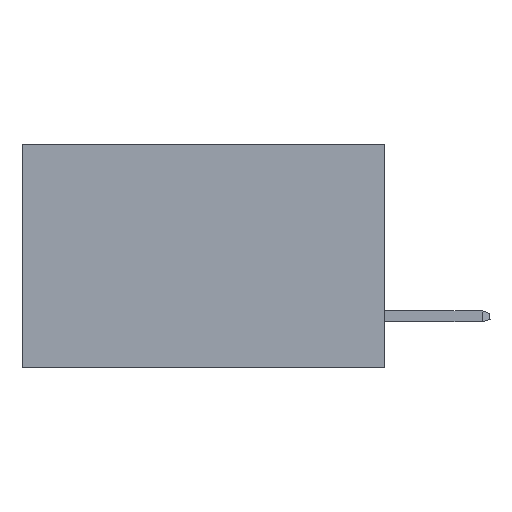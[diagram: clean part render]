
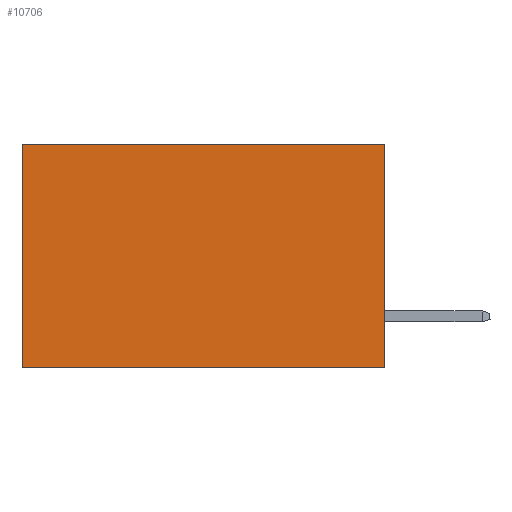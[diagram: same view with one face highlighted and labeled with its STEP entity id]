
A CAD part, left-side view. The second image highlights one B-rep face of the part: STEP entity #10706.
In plain terms, the highlighted planar face has unit normal (-1, 0, 0).
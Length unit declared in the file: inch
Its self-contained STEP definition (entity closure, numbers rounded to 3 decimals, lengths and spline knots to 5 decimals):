
#26 = CARTESIAN_POINT ( 'NONE',  ( 0.298, 0., 0. ) ) ;
#44 = EDGE_CURVE ( 'NONE', #19193, #22223, #3596, .T. ) ;
#255 = ORIENTED_EDGE ( 'NONE', *, *, #44, .F. ) ;
#314 = LINE ( 'NONE', #17905, #12894 ) ;
#651 = ORIENTED_EDGE ( 'NONE', *, *, #15813, .F. ) ;
#1596 = DIRECTION ( 'NONE',  ( 0., 0., -1. ) ) ;
#1837 = CARTESIAN_POINT ( 'NONE',  ( 0.298, 0., 0. ) ) ;
#3596 = LINE ( 'NONE', #26, #14363 ) ;
#5618 = DIRECTION ( 'NONE',  ( 0., 0., -1. ) ) ;
#6966 = VERTEX_POINT ( 'NONE', #21133 ) ;
#9540 = LINE ( 'NONE', #19866, #18079 ) ;
#10523 = EDGE_CURVE ( 'NONE', #19193, #14142, #9540, .T. ) ;
#10706 = ADVANCED_FACE ( 'NONE', ( #13895 ), #16666, .F. ) ;
#12894 = VECTOR ( 'NONE', #21604, 39.37008 ) ;
#13228 = EDGE_LOOP ( 'NONE', ( #19385, #651, #255, #17297 ) ) ;
#13699 = LINE ( 'NONE', #14553, #16409 ) ;
#13895 = FACE_OUTER_BOUND ( 'NONE', #13228, .T. ) ;
#13957 = CARTESIAN_POINT ( 'NONE',  ( 0.298, 0.6, 0. ) ) ;
#14142 = VERTEX_POINT ( 'NONE', #13957 ) ;
#14231 = DIRECTION ( 'NONE',  ( 0., 1., 0. ) ) ;
#14307 = CARTESIAN_POINT ( 'NONE',  ( 0.298, 0., -0.37 ) ) ;
#14363 = VECTOR ( 'NONE', #5618, 39.37008 ) ;
#14553 = CARTESIAN_POINT ( 'NONE',  ( 0.298, 0., -0.37 ) ) ;
#14811 = DIRECTION ( 'NONE',  ( 1., 0., 0. ) ) ;
#15813 = EDGE_CURVE ( 'NONE', #22223, #6966, #13699, .T. ) ;
#16409 = VECTOR ( 'NONE', #20272, 39.37008 ) ;
#16666 = PLANE ( 'NONE',  #18188 ) ;
#17297 = ORIENTED_EDGE ( 'NONE', *, *, #10523, .T. ) ;
#17905 = CARTESIAN_POINT ( 'NONE',  ( 0.298, 0.6, 0. ) ) ;
#18079 = VECTOR ( 'NONE', #14231, 39.37008 ) ;
#18188 = AXIS2_PLACEMENT_3D ( 'NONE', #1837, #14811, #1596 ) ;
#18392 = CARTESIAN_POINT ( 'NONE',  ( 0.298, 0., 0. ) ) ;
#19193 = VERTEX_POINT ( 'NONE', #18392 ) ;
#19385 = ORIENTED_EDGE ( 'NONE', *, *, #20311, .T. ) ;
#19866 = CARTESIAN_POINT ( 'NONE',  ( 0.298, 0., 0. ) ) ;
#20272 = DIRECTION ( 'NONE',  ( 0., 1., 0. ) ) ;
#20311 = EDGE_CURVE ( 'NONE', #14142, #6966, #314, .T. ) ;
#21133 = CARTESIAN_POINT ( 'NONE',  ( 0.298, 0.6, -0.37 ) ) ;
#21604 = DIRECTION ( 'NONE',  ( 0., 0., -1. ) ) ;
#22223 = VERTEX_POINT ( 'NONE', #14307 ) ;
